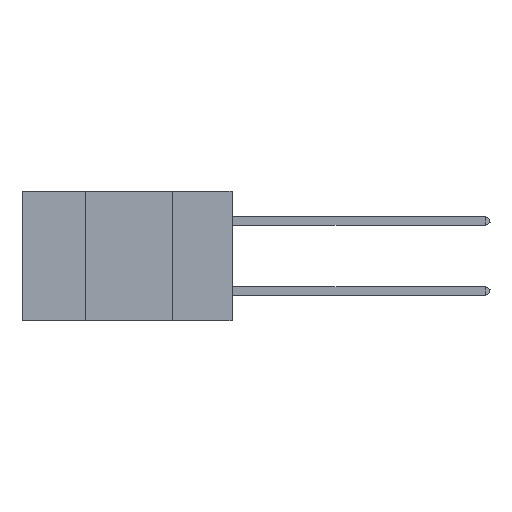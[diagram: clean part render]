
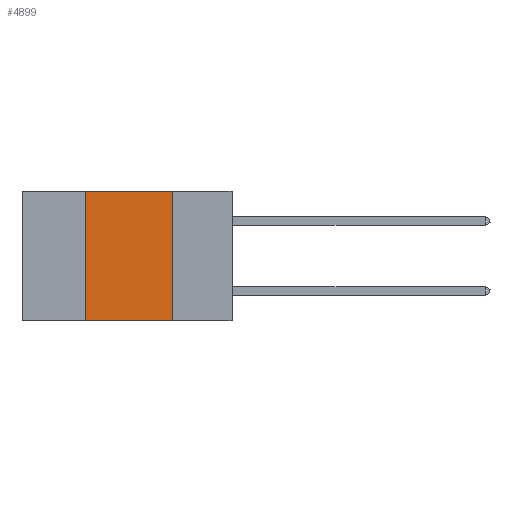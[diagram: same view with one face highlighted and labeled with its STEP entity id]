
A CAD part, left-side view. The second image highlights one B-rep face of the part: STEP entity #4899.
In plain terms, the highlighted planar face has unit normal (-1, 0, 0).
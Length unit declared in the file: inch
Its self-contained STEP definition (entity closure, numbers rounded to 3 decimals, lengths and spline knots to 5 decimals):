
#53 = VERTEX_POINT ( 'NONE', #3336 ) ;
#262 = LINE ( 'NONE', #4515, #2744 ) ;
#462 = ORIENTED_EDGE ( 'NONE', *, *, #8394, .F. ) ;
#938 = VERTEX_POINT ( 'NONE', #8766 ) ;
#947 = DIRECTION ( 'NONE',  ( 1., 0., 0. ) ) ;
#1572 = LINE ( 'NONE', #5836, #7552 ) ;
#2031 = PLANE ( 'NONE',  #5995 ) ;
#2079 = EDGE_CURVE ( 'NONE', #9147, #938, #262, .T. ) ;
#2317 = FACE_OUTER_BOUND ( 'NONE', #2721, .T. ) ;
#2518 = VECTOR ( 'NONE', #5590, 39.37008 ) ;
#2721 = EDGE_LOOP ( 'NONE', ( #462, #8331, #4535, #9631 ) ) ;
#2744 = VECTOR ( 'NONE', #7151, 39.37008 ) ;
#3336 = CARTESIAN_POINT ( 'NONE',  ( 0., 0.17, -0.37 ) ) ;
#3471 = EDGE_CURVE ( 'NONE', #9534, #53, #1572, .T. ) ;
#3884 = DIRECTION ( 'NONE',  ( 0., 0., 1. ) ) ;
#3976 = DIRECTION ( 'NONE',  ( 0., -1., 0. ) ) ;
#4515 = CARTESIAN_POINT ( 'NONE',  ( 0., 0.6, 0. ) ) ;
#4535 = ORIENTED_EDGE ( 'NONE', *, *, #6921, .F. ) ;
#4688 = CARTESIAN_POINT ( 'NONE',  ( 0., 0.42, 0. ) ) ;
#4803 = CARTESIAN_POINT ( 'NONE',  ( 0., 0.17, 0. ) ) ;
#4899 = ADVANCED_FACE ( 'NONE', ( #2317 ), #2031, .F. ) ;
#5378 = CARTESIAN_POINT ( 'NONE',  ( 0., 0.6, 0. ) ) ;
#5590 = DIRECTION ( 'NONE',  ( 0., 0., -1. ) ) ;
#5836 = CARTESIAN_POINT ( 'NONE',  ( 0., 0.6, -0.37 ) ) ;
#5995 = AXIS2_PLACEMENT_3D ( 'NONE', #5378, #947, #7776 ) ;
#6921 = EDGE_CURVE ( 'NONE', #9534, #9147, #7254, .T. ) ;
#7151 = DIRECTION ( 'NONE',  ( 0., -1., 0. ) ) ;
#7254 = LINE ( 'NONE', #4688, #8798 ) ;
#7552 = VECTOR ( 'NONE', #3976, 39.37008 ) ;
#7776 = DIRECTION ( 'NONE',  ( 0., 0., -1. ) ) ;
#8230 = CARTESIAN_POINT ( 'NONE',  ( 0., 0.42, 0. ) ) ;
#8331 = ORIENTED_EDGE ( 'NONE', *, *, #2079, .F. ) ;
#8394 = EDGE_CURVE ( 'NONE', #938, #53, #8429, .T. ) ;
#8429 = LINE ( 'NONE', #4803, #2518 ) ;
#8766 = CARTESIAN_POINT ( 'NONE',  ( 0., 0.17, 0. ) ) ;
#8798 = VECTOR ( 'NONE', #3884, 39.37008 ) ;
#9113 = CARTESIAN_POINT ( 'NONE',  ( 0., 0.42, -0.37 ) ) ;
#9147 = VERTEX_POINT ( 'NONE', #8230 ) ;
#9534 = VERTEX_POINT ( 'NONE', #9113 ) ;
#9631 = ORIENTED_EDGE ( 'NONE', *, *, #3471, .T. ) ;
